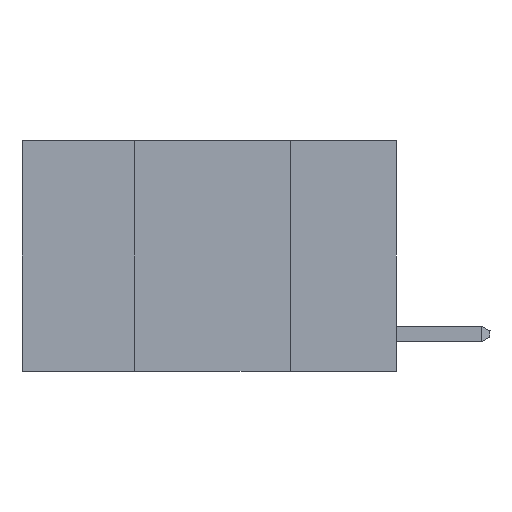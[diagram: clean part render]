
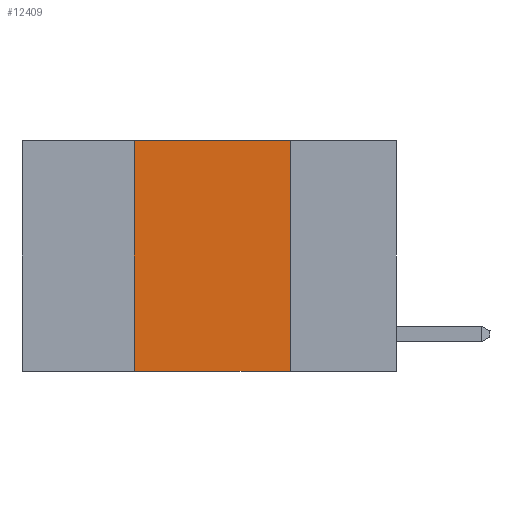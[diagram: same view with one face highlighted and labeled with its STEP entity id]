
A CAD part, left-side view. The second image highlights one B-rep face of the part: STEP entity #12409.
In plain terms, the highlighted planar face has unit normal (-1, 0, 0).
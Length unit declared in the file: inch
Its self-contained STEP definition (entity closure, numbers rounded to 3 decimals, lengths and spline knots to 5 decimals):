
#793 = CARTESIAN_POINT ( 'NONE',  ( 0., 0.42, 0. ) ) ;
#1256 = VERTEX_POINT ( 'NONE', #5977 ) ;
#2921 = LINE ( 'NONE', #17185, #7853 ) ;
#3407 = EDGE_CURVE ( 'NONE', #16906, #1256, #19728, .T. ) ;
#5278 = EDGE_CURVE ( 'NONE', #14752, #7935, #13276, .T. ) ;
#5977 = CARTESIAN_POINT ( 'NONE',  ( 0., 0.17, -0.37 ) ) ;
#6101 = DIRECTION ( 'NONE',  ( 0., -1., 0. ) ) ;
#6723 = FACE_OUTER_BOUND ( 'NONE', #15586, .T. ) ;
#7046 = EDGE_CURVE ( 'NONE', #16906, #14752, #12976, .T. ) ;
#7853 = VECTOR ( 'NONE', #15590, 39.37008 ) ;
#7935 = VERTEX_POINT ( 'NONE', #18688 ) ;
#9133 = CARTESIAN_POINT ( 'NONE',  ( 0., 0.6, 0. ) ) ;
#9239 = ORIENTED_EDGE ( 'NONE', *, *, #9816, .F. ) ;
#9637 = CARTESIAN_POINT ( 'NONE',  ( 0., 0.6, -0.37 ) ) ;
#9816 = EDGE_CURVE ( 'NONE', #7935, #1256, #2921, .T. ) ;
#11053 = ORIENTED_EDGE ( 'NONE', *, *, #7046, .F. ) ;
#11924 = PLANE ( 'NONE',  #20246 ) ;
#12409 = ADVANCED_FACE ( 'NONE', ( #6723 ), #11924, .F. ) ;
#12601 = VECTOR ( 'NONE', #16451, 39.37008 ) ;
#12613 = DIRECTION ( 'NONE',  ( 0., 0., 1. ) ) ;
#12976 = LINE ( 'NONE', #793, #14582 ) ;
#13276 = LINE ( 'NONE', #14341, #17203 ) ;
#13689 = ORIENTED_EDGE ( 'NONE', *, *, #3407, .T. ) ;
#14341 = CARTESIAN_POINT ( 'NONE',  ( 0., 0.6, 0. ) ) ;
#14582 = VECTOR ( 'NONE', #12613, 39.37008 ) ;
#14752 = VERTEX_POINT ( 'NONE', #20473 ) ;
#15586 = EDGE_LOOP ( 'NONE', ( #9239, #16933, #11053, #13689 ) ) ;
#15590 = DIRECTION ( 'NONE',  ( 0., 0., -1. ) ) ;
#16451 = DIRECTION ( 'NONE',  ( 0., -1., 0. ) ) ;
#16873 = DIRECTION ( 'NONE',  ( 0., 0., -1. ) ) ;
#16906 = VERTEX_POINT ( 'NONE', #20988 ) ;
#16933 = ORIENTED_EDGE ( 'NONE', *, *, #5278, .F. ) ;
#17185 = CARTESIAN_POINT ( 'NONE',  ( 0., 0.17, 0. ) ) ;
#17203 = VECTOR ( 'NONE', #6101, 39.37008 ) ;
#18688 = CARTESIAN_POINT ( 'NONE',  ( 0., 0.17, 0. ) ) ;
#19728 = LINE ( 'NONE', #9637, #12601 ) ;
#20246 = AXIS2_PLACEMENT_3D ( 'NONE', #9133, #20327, #16873 ) ;
#20327 = DIRECTION ( 'NONE',  ( 1., 0., 0. ) ) ;
#20473 = CARTESIAN_POINT ( 'NONE',  ( 0., 0.42, 0. ) ) ;
#20988 = CARTESIAN_POINT ( 'NONE',  ( 0., 0.42, -0.37 ) ) ;
